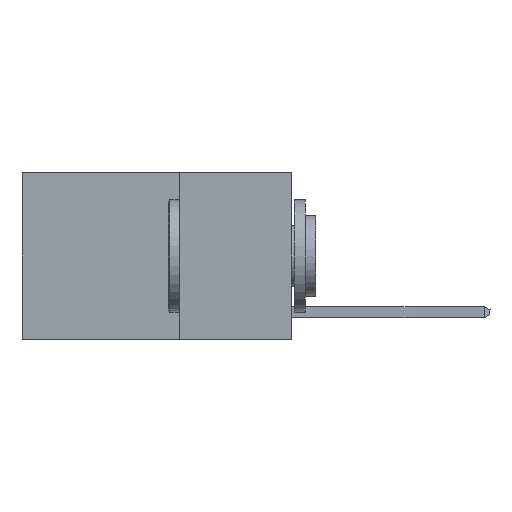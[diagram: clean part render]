
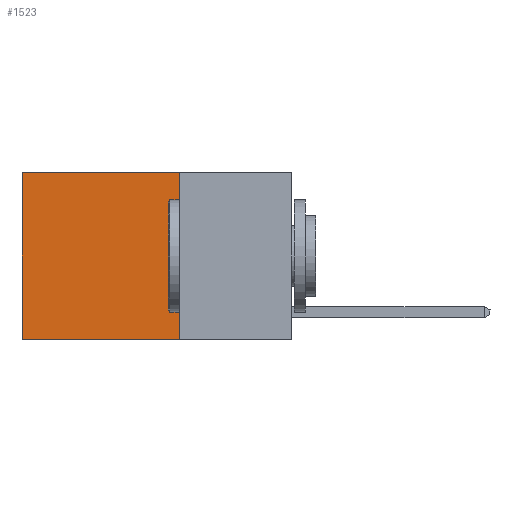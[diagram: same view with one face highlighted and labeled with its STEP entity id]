
A CAD part, left-side view. The second image highlights one B-rep face of the part: STEP entity #1523.
In plain terms, the highlighted planar face has unit normal (-1, 0, 0).
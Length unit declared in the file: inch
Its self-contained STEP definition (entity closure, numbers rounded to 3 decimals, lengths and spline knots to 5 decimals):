
#1001 = VERTEX_POINT ( 'NONE', #16986 ) ;
#1350 = VECTOR ( 'NONE', #11705, 39.37008 ) ;
#1523 = ADVANCED_FACE ( 'NONE', ( #8524 ), #16083, .F. ) ;
#1817 = CARTESIAN_POINT ( 'NONE',  ( 0.2625, 0.6, 0. ) ) ;
#1929 = LINE ( 'NONE', #6639, #17130 ) ;
#1994 = VERTEX_POINT ( 'NONE', #12060 ) ;
#3223 = DIRECTION ( 'NONE',  ( 0., 0., -1. ) ) ;
#3523 = ORIENTED_EDGE ( 'NONE', *, *, #3929, .T. ) ;
#3868 = ORIENTED_EDGE ( 'NONE', *, *, #16381, .F. ) ;
#3929 = EDGE_CURVE ( 'NONE', #1994, #1001, #9975, .T. ) ;
#5534 = CARTESIAN_POINT ( 'NONE',  ( 0.2625, 0.25, 0. ) ) ;
#6639 = CARTESIAN_POINT ( 'NONE',  ( 0.2625, 0.25, -0.37 ) ) ;
#6945 = VERTEX_POINT ( 'NONE', #17573 ) ;
#7613 = LINE ( 'NONE', #11644, #1350 ) ;
#7827 = AXIS2_PLACEMENT_3D ( 'NONE', #9214, #14791, #9277 ) ;
#8312 = VERTEX_POINT ( 'NONE', #15282 ) ;
#8524 = FACE_OUTER_BOUND ( 'NONE', #16517, .T. ) ;
#9214 = CARTESIAN_POINT ( 'NONE',  ( 0.2625, 0.25, 0. ) ) ;
#9277 = DIRECTION ( 'NONE',  ( 0., 0., -1. ) ) ;
#9975 = LINE ( 'NONE', #1817, #11284 ) ;
#11284 = VECTOR ( 'NONE', #3223, 39.37008 ) ;
#11528 = EDGE_CURVE ( 'NONE', #6945, #1994, #17157, .T. ) ;
#11644 = CARTESIAN_POINT ( 'NONE',  ( 0.2625, 0.25, 0. ) ) ;
#11705 = DIRECTION ( 'NONE',  ( 0., 0., -1. ) ) ;
#12060 = CARTESIAN_POINT ( 'NONE',  ( 0.2625, 0.6, 0. ) ) ;
#12096 = EDGE_CURVE ( 'NONE', #8312, #1001, #1929, .T. ) ;
#12230 = DIRECTION ( 'NONE',  ( 0., 1., 0. ) ) ;
#13055 = ORIENTED_EDGE ( 'NONE', *, *, #12096, .F. ) ;
#14014 = DIRECTION ( 'NONE',  ( 0., 1., 0. ) ) ;
#14791 = DIRECTION ( 'NONE',  ( 1., 0., 0. ) ) ;
#14979 = ORIENTED_EDGE ( 'NONE', *, *, #11528, .T. ) ;
#15282 = CARTESIAN_POINT ( 'NONE',  ( 0.2625, 0.25, -0.37 ) ) ;
#15378 = VECTOR ( 'NONE', #14014, 39.37008 ) ;
#16083 = PLANE ( 'NONE',  #7827 ) ;
#16381 = EDGE_CURVE ( 'NONE', #6945, #8312, #7613, .T. ) ;
#16517 = EDGE_LOOP ( 'NONE', ( #3523, #13055, #3868, #14979 ) ) ;
#16986 = CARTESIAN_POINT ( 'NONE',  ( 0.2625, 0.6, -0.37 ) ) ;
#17130 = VECTOR ( 'NONE', #12230, 39.37008 ) ;
#17157 = LINE ( 'NONE', #5534, #15378 ) ;
#17573 = CARTESIAN_POINT ( 'NONE',  ( 0.2625, 0.25, 0. ) ) ;
